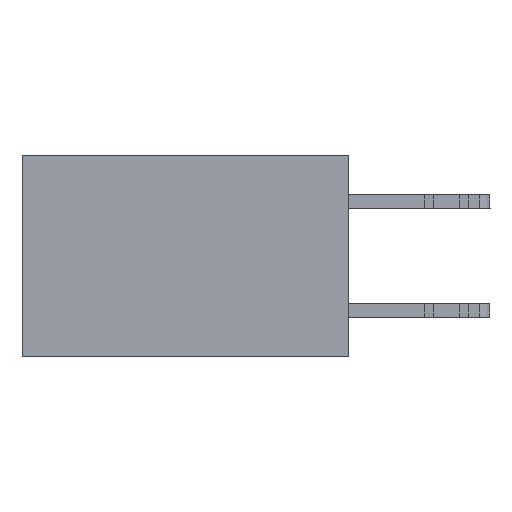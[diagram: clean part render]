
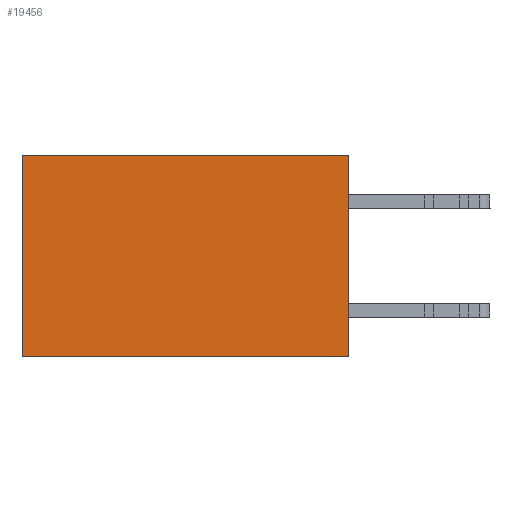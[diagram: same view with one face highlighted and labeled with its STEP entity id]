
A CAD part, left-side view. The second image highlights one B-rep face of the part: STEP entity #19456.
In plain terms, the highlighted planar face has unit normal (-1, 0, 0).
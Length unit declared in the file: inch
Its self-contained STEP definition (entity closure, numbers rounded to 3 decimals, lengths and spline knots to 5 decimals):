
#728 = LINE ( 'NONE', #17501, #14229 ) ;
#1656 = EDGE_CURVE ( 'NONE', #18089, #4642, #30277, .T. ) ;
#2058 = CARTESIAN_POINT ( 'NONE',  ( 0.298, 0., -0.37 ) ) ;
#2129 = EDGE_CURVE ( 'NONE', #25020, #11980, #728, .T. ) ;
#3963 = DIRECTION ( 'NONE',  ( 0., 1., 0. ) ) ;
#4642 = VERTEX_POINT ( 'NONE', #2058 ) ;
#5640 = ORIENTED_EDGE ( 'NONE', *, *, #7311, .T. ) ;
#5794 = DIRECTION ( 'NONE',  ( 0., 1., 0. ) ) ;
#6073 = CARTESIAN_POINT ( 'NONE',  ( 0.298, 0.6, -0.37 ) ) ;
#7311 = EDGE_CURVE ( 'NONE', #18089, #25020, #15376, .T. ) ;
#7492 = VECTOR ( 'NONE', #3963, 39.37008 ) ;
#8451 = ORIENTED_EDGE ( 'NONE', *, *, #29836, .F. ) ;
#11980 = VERTEX_POINT ( 'NONE', #6073 ) ;
#12431 = ORIENTED_EDGE ( 'NONE', *, *, #1656, .F. ) ;
#14229 = VECTOR ( 'NONE', #24430, 39.37008 ) ;
#14332 = CARTESIAN_POINT ( 'NONE',  ( 0.298, 0., 0. ) ) ;
#14968 = VECTOR ( 'NONE', #5794, 39.37008 ) ;
#15376 = LINE ( 'NONE', #15852, #7492 ) ;
#15627 = AXIS2_PLACEMENT_3D ( 'NONE', #19434, #18999, #16433 ) ;
#15852 = CARTESIAN_POINT ( 'NONE',  ( 0.298, 0., 0. ) ) ;
#16433 = DIRECTION ( 'NONE',  ( 0., 0., -1. ) ) ;
#17082 = PLANE ( 'NONE',  #15627 ) ;
#17501 = CARTESIAN_POINT ( 'NONE',  ( 0.298, 0.6, 0. ) ) ;
#17676 = ORIENTED_EDGE ( 'NONE', *, *, #2129, .T. ) ;
#18089 = VERTEX_POINT ( 'NONE', #25808 ) ;
#18999 = DIRECTION ( 'NONE',  ( 1., 0., 0. ) ) ;
#19434 = CARTESIAN_POINT ( 'NONE',  ( 0.298, 0., 0. ) ) ;
#19456 = ADVANCED_FACE ( 'NONE', ( #28399 ), #17082, .F. ) ;
#21017 = DIRECTION ( 'NONE',  ( 0., 0., -1. ) ) ;
#24430 = DIRECTION ( 'NONE',  ( 0., 0., -1. ) ) ;
#25020 = VERTEX_POINT ( 'NONE', #28658 ) ;
#25808 = CARTESIAN_POINT ( 'NONE',  ( 0.298, 0., 0. ) ) ;
#27082 = CARTESIAN_POINT ( 'NONE',  ( 0.298, 0., -0.37 ) ) ;
#27596 = LINE ( 'NONE', #27082, #14968 ) ;
#27971 = EDGE_LOOP ( 'NONE', ( #17676, #8451, #12431, #5640 ) ) ;
#28399 = FACE_OUTER_BOUND ( 'NONE', #27971, .T. ) ;
#28425 = VECTOR ( 'NONE', #21017, 39.37008 ) ;
#28658 = CARTESIAN_POINT ( 'NONE',  ( 0.298, 0.6, 0. ) ) ;
#29836 = EDGE_CURVE ( 'NONE', #4642, #11980, #27596, .T. ) ;
#30277 = LINE ( 'NONE', #14332, #28425 ) ;
